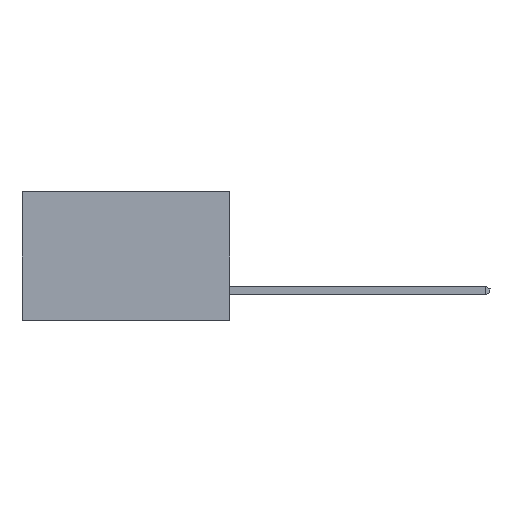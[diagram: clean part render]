
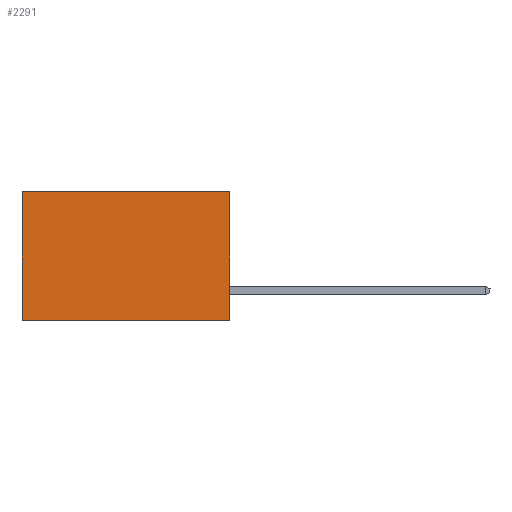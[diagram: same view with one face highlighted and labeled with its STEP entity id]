
A CAD part, left-side view. The second image highlights one B-rep face of the part: STEP entity #2291.
In plain terms, the highlighted planar face has unit normal (-1, 0, 0).
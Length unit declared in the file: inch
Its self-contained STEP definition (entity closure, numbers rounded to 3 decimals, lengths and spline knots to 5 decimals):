
#292 = ORIENTED_EDGE ( 'NONE', *, *, #3465, .T. ) ;
#368 = VECTOR ( 'NONE', #5804, 39.37008 ) ;
#1257 = CARTESIAN_POINT ( 'NONE',  ( 0.2615, 0., 0. ) ) ;
#1452 = EDGE_CURVE ( 'NONE', #6880, #7739, #8839, .T. ) ;
#1471 = VECTOR ( 'NONE', #1519, 39.37008 ) ;
#1519 = DIRECTION ( 'NONE',  ( 0., 0., -1. ) ) ;
#1790 = CARTESIAN_POINT ( 'NONE',  ( 0.2615, 0., -0.37 ) ) ;
#2291 = ADVANCED_FACE ( 'NONE', ( #2389 ), #3103, .F. ) ;
#2366 = LINE ( 'NONE', #9368, #9858 ) ;
#2389 = FACE_OUTER_BOUND ( 'NONE', #9073, .T. ) ;
#2537 = EDGE_CURVE ( 'NONE', #8093, #6880, #2366, .T. ) ;
#2608 = CARTESIAN_POINT ( 'NONE',  ( 0.2615, 0.6, -0.37 ) ) ;
#2784 = CARTESIAN_POINT ( 'NONE',  ( 0.2615, 0.6, 0. ) ) ;
#3054 = AXIS2_PLACEMENT_3D ( 'NONE', #7958, #7176, #3914 ) ;
#3103 = PLANE ( 'NONE',  #3054 ) ;
#3268 = EDGE_CURVE ( 'NONE', #4367, #7739, #7683, .T. ) ;
#3295 = ORIENTED_EDGE ( 'NONE', *, *, #1452, .F. ) ;
#3465 = EDGE_CURVE ( 'NONE', #8093, #4367, #9026, .T. ) ;
#3914 = DIRECTION ( 'NONE',  ( 0., 0., -1. ) ) ;
#4085 = ORIENTED_EDGE ( 'NONE', *, *, #2537, .F. ) ;
#4110 = DIRECTION ( 'NONE',  ( 0., 1., 0. ) ) ;
#4311 = CARTESIAN_POINT ( 'NONE',  ( 0.2615, 0., -0.37 ) ) ;
#4367 = VERTEX_POINT ( 'NONE', #2784 ) ;
#5804 = DIRECTION ( 'NONE',  ( 0., 1., 0. ) ) ;
#6259 = VECTOR ( 'NONE', #4110, 39.37008 ) ;
#6880 = VERTEX_POINT ( 'NONE', #1790 ) ;
#7032 = DIRECTION ( 'NONE',  ( 0., 0., -1. ) ) ;
#7176 = DIRECTION ( 'NONE',  ( 1., 0., 0. ) ) ;
#7683 = LINE ( 'NONE', #9378, #1471 ) ;
#7739 = VERTEX_POINT ( 'NONE', #2608 ) ;
#7958 = CARTESIAN_POINT ( 'NONE',  ( 0.2615, 0., -0.37 ) ) ;
#8093 = VERTEX_POINT ( 'NONE', #9407 ) ;
#8839 = LINE ( 'NONE', #4311, #6259 ) ;
#9026 = LINE ( 'NONE', #1257, #368 ) ;
#9031 = ORIENTED_EDGE ( 'NONE', *, *, #3268, .T. ) ;
#9073 = EDGE_LOOP ( 'NONE', ( #9031, #3295, #4085, #292 ) ) ;
#9368 = CARTESIAN_POINT ( 'NONE',  ( 0.2615, 0., -0.37 ) ) ;
#9378 = CARTESIAN_POINT ( 'NONE',  ( 0.2615, 0.6, -0.37 ) ) ;
#9407 = CARTESIAN_POINT ( 'NONE',  ( 0.2615, 0., 0. ) ) ;
#9858 = VECTOR ( 'NONE', #7032, 39.37008 ) ;
